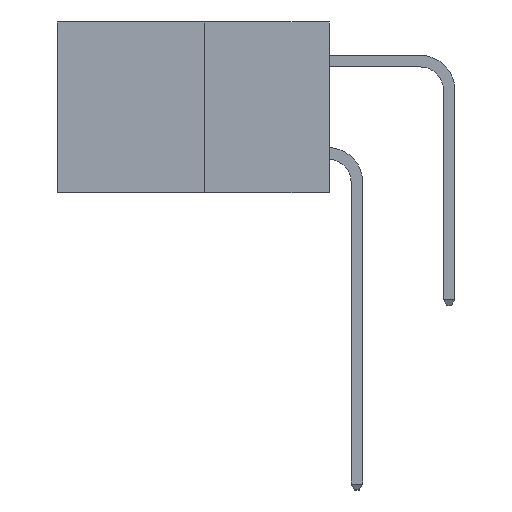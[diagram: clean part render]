
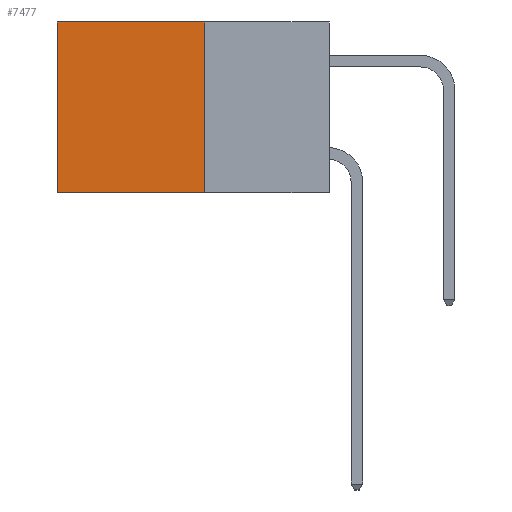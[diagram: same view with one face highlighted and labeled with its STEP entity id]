
A CAD part, left-side view. The second image highlights one B-rep face of the part: STEP entity #7477.
In plain terms, the highlighted planar face has unit normal (-1, 0, 0).
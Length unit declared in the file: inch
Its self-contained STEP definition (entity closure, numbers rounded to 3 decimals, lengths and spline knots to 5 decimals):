
#117 = CARTESIAN_POINT ( 'NONE',  ( 0.277, 0.27, 0. ) ) ;
#217 = EDGE_CURVE ( 'NONE', #813, #10452, #1267, .T. ) ;
#680 = EDGE_CURVE ( 'NONE', #6507, #2012, #4860, .T. ) ;
#768 = CARTESIAN_POINT ( 'NONE',  ( 0.277, 0.59, -0.37 ) ) ;
#813 = VERTEX_POINT ( 'NONE', #7789 ) ;
#1267 = LINE ( 'NONE', #6131, #7396 ) ;
#1517 = ORIENTED_EDGE ( 'NONE', *, *, #4646, .F. ) ;
#1875 = CARTESIAN_POINT ( 'NONE',  ( 0.277, 0.59, -0.37 ) ) ;
#2012 = VERTEX_POINT ( 'NONE', #8241 ) ;
#2491 = DIRECTION ( 'NONE',  ( 0., 0., -1. ) ) ;
#2818 = DIRECTION ( 'NONE',  ( 0., 0., -1. ) ) ;
#3119 = LINE ( 'NONE', #1875, #7353 ) ;
#3293 = CARTESIAN_POINT ( 'NONE',  ( 0.277, 0.27, -0.37 ) ) ;
#3614 = CARTESIAN_POINT ( 'NONE',  ( 0.277, 0.27, -0.37 ) ) ;
#3617 = EDGE_LOOP ( 'NONE', ( #5013, #10622, #1517, #8744 ) ) ;
#4142 = CARTESIAN_POINT ( 'NONE',  ( 0.277, 0.27, 0. ) ) ;
#4646 = EDGE_CURVE ( 'NONE', #6507, #813, #9338, .T. ) ;
#4860 = LINE ( 'NONE', #117, #9624 ) ;
#5013 = ORIENTED_EDGE ( 'NONE', *, *, #6676, .T. ) ;
#6131 = CARTESIAN_POINT ( 'NONE',  ( 0.277, 0.27, -0.37 ) ) ;
#6172 = PLANE ( 'NONE',  #7970 ) ;
#6269 = DIRECTION ( 'NONE',  ( 0., 1., 0. ) ) ;
#6507 = VERTEX_POINT ( 'NONE', #4142 ) ;
#6676 = EDGE_CURVE ( 'NONE', #2012, #10452, #3119, .T. ) ;
#7132 = VECTOR ( 'NONE', #2491, 39.37008 ) ;
#7353 = VECTOR ( 'NONE', #9435, 39.37008 ) ;
#7396 = VECTOR ( 'NONE', #6269, 39.37008 ) ;
#7477 = ADVANCED_FACE ( 'NONE', ( #10357 ), #6172, .F. ) ;
#7596 = DIRECTION ( 'NONE',  ( 0., 1., 0. ) ) ;
#7789 = CARTESIAN_POINT ( 'NONE',  ( 0.277, 0.27, -0.37 ) ) ;
#7865 = DIRECTION ( 'NONE',  ( 1., 0., 0. ) ) ;
#7970 = AXIS2_PLACEMENT_3D ( 'NONE', #3614, #7865, #2818 ) ;
#8241 = CARTESIAN_POINT ( 'NONE',  ( 0.277, 0.59, 0. ) ) ;
#8744 = ORIENTED_EDGE ( 'NONE', *, *, #680, .T. ) ;
#9338 = LINE ( 'NONE', #3293, #7132 ) ;
#9435 = DIRECTION ( 'NONE',  ( 0., 0., -1. ) ) ;
#9624 = VECTOR ( 'NONE', #7596, 39.37008 ) ;
#10357 = FACE_OUTER_BOUND ( 'NONE', #3617, .T. ) ;
#10452 = VERTEX_POINT ( 'NONE', #768 ) ;
#10622 = ORIENTED_EDGE ( 'NONE', *, *, #217, .F. ) ;
